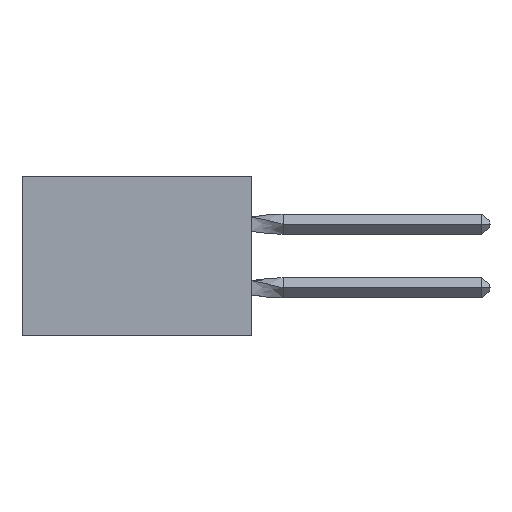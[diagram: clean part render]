
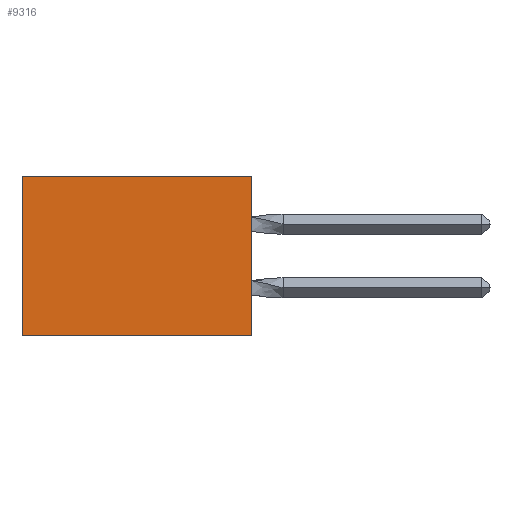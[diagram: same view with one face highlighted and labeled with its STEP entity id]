
A CAD part, left-side view. The second image highlights one B-rep face of the part: STEP entity #9316.
In plain terms, the highlighted planar face has unit normal (-1, 0, 0).
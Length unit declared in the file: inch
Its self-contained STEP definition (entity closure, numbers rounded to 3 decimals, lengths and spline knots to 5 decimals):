
#15 = EDGE_CURVE ( 'NONE', #26121, #889, #5445, .T. ) ;
#129 = CARTESIAN_POINT ( 'NONE',  ( 0.305, 0., -0.5 ) ) ;
#725 = VECTOR ( 'NONE', #29900, 39.37008 ) ;
#889 = VERTEX_POINT ( 'NONE', #8516 ) ;
#1018 = FACE_OUTER_BOUND ( 'NONE', #22124, .T. ) ;
#1025 = VECTOR ( 'NONE', #26703, 39.37008 ) ;
#1507 = ORIENTED_EDGE ( 'NONE', *, *, #14099, .T. ) ;
#2350 = ORIENTED_EDGE ( 'NONE', *, *, #15, .T. ) ;
#3531 = VERTEX_POINT ( 'NONE', #25481 ) ;
#3855 = EDGE_CURVE ( 'NONE', #3531, #4635, #31270, .T. ) ;
#4303 = AXIS2_PLACEMENT_3D ( 'NONE', #24964, #24741, #27183 ) ;
#4635 = VERTEX_POINT ( 'NONE', #31307 ) ;
#4673 = CARTESIAN_POINT ( 'NONE',  ( 0.305, 0.72, -0.5 ) ) ;
#4982 = DIRECTION ( 'NONE',  ( 0., 0., -1. ) ) ;
#5445 = LINE ( 'NONE', #4673, #27534 ) ;
#5635 = LINE ( 'NONE', #10441, #725 ) ;
#7440 = LINE ( 'NONE', #12356, #1025 ) ;
#8516 = CARTESIAN_POINT ( 'NONE',  ( 0.305, 0.72, -0.5 ) ) ;
#8940 = ORIENTED_EDGE ( 'NONE', *, *, #22690, .F. ) ;
#9316 = ADVANCED_FACE ( 'NONE', ( #1018 ), #17200, .F. ) ;
#10441 = CARTESIAN_POINT ( 'NONE',  ( 0.305, 0., 0. ) ) ;
#12356 = CARTESIAN_POINT ( 'NONE',  ( 0.305, 0., -0.5 ) ) ;
#14099 = EDGE_CURVE ( 'NONE', #3531, #26121, #5635, .T. ) ;
#14888 = CARTESIAN_POINT ( 'NONE',  ( 0.305, 0.72, 0. ) ) ;
#17200 = PLANE ( 'NONE',  #4303 ) ;
#22124 = EDGE_LOOP ( 'NONE', ( #2350, #8940, #30816, #1507 ) ) ;
#22690 = EDGE_CURVE ( 'NONE', #4635, #889, #7440, .T. ) ;
#24741 = DIRECTION ( 'NONE',  ( 1., 0., 0. ) ) ;
#24964 = CARTESIAN_POINT ( 'NONE',  ( 0.305, 0., -0.5 ) ) ;
#25481 = CARTESIAN_POINT ( 'NONE',  ( 0.305, 0., 0. ) ) ;
#25545 = VECTOR ( 'NONE', #29181, 39.37008 ) ;
#26121 = VERTEX_POINT ( 'NONE', #14888 ) ;
#26703 = DIRECTION ( 'NONE',  ( 0., 1., 0. ) ) ;
#27183 = DIRECTION ( 'NONE',  ( 0., 0., -1. ) ) ;
#27534 = VECTOR ( 'NONE', #4982, 39.37008 ) ;
#29181 = DIRECTION ( 'NONE',  ( 0., 0., -1. ) ) ;
#29900 = DIRECTION ( 'NONE',  ( 0., 1., 0. ) ) ;
#30816 = ORIENTED_EDGE ( 'NONE', *, *, #3855, .F. ) ;
#31270 = LINE ( 'NONE', #129, #25545 ) ;
#31307 = CARTESIAN_POINT ( 'NONE',  ( 0.305, 0., -0.5 ) ) ;
